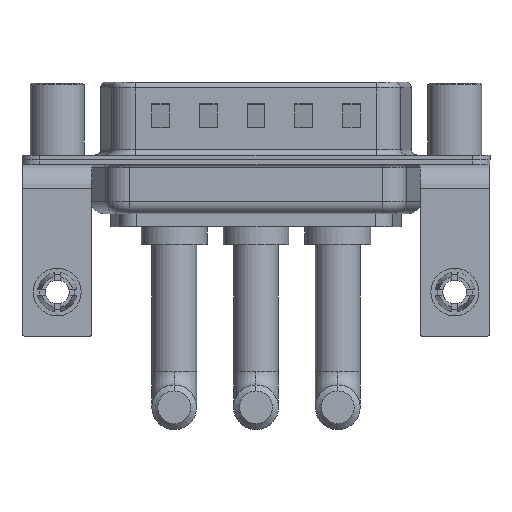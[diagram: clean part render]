
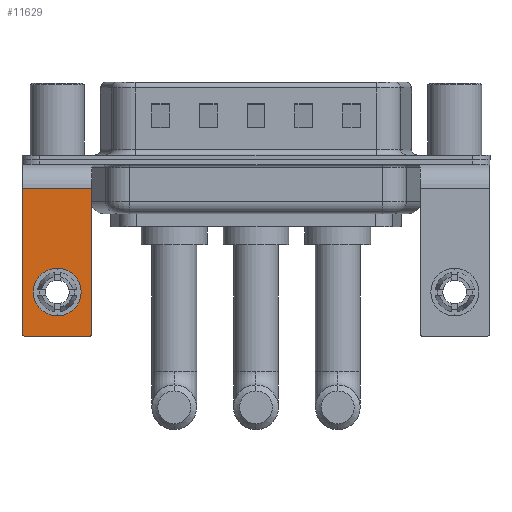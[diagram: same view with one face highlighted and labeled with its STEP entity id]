
A CAD part, front view. The second image highlights one B-rep face of the part: STEP entity #11629.
In plain terms, the highlighted planar face has unit normal (0, -1, 0).
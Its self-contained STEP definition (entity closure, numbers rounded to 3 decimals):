
#14 = ORIENTED_EDGE ( 'NONE', *, *, #4741, .T. ) ;
#195 = CARTESIAN_POINT ( 'NONE',  ( -2.9, -6.25, -2.4 ) ) ;
#734 = VERTEX_POINT ( 'NONE', #4127 ) ;
#1014 = DIRECTION ( 'NONE',  ( 0., 0., -1. ) ) ;
#1073 = CARTESIAN_POINT ( 'NONE',  ( 2.65, -6.25, -14.55 ) ) ;
#1187 = ORIENTED_EDGE ( 'NONE', *, *, #3510, .T. ) ;
#1225 = CIRCLE ( 'NONE', #14565, 2. ) ;
#1451 = EDGE_LOOP ( 'NONE', ( #7569, #5173, #8265, #14, #3821, #8792 ) ) ;
#1598 = DIRECTION ( 'NONE',  ( 0., 1., 0. ) ) ;
#1828 = AXIS2_PLACEMENT_3D ( 'NONE', #2882, #14920, #13556 ) ;
#2653 = EDGE_CURVE ( 'NONE', #9463, #10785, #3996, .T. ) ;
#2752 = VECTOR ( 'NONE', #1014, 1000. ) ;
#2882 = CARTESIAN_POINT ( 'NONE',  ( -2.65, -6.25, -14.55 ) ) ;
#2941 = ORIENTED_EDGE ( 'NONE', *, *, #8147, .T. ) ;
#3287 = DIRECTION ( 'NONE',  ( 0., 0., 1. ) ) ;
#3510 = EDGE_CURVE ( 'NONE', #17555, #18703, #1225, .T. ) ;
#3821 = ORIENTED_EDGE ( 'NONE', *, *, #11553, .F. ) ;
#3996 = CIRCLE ( 'NONE', #1828, 0.25 ) ;
#4127 = CARTESIAN_POINT ( 'NONE',  ( -2.9, -6.25, -2.4 ) ) ;
#4329 = AXIS2_PLACEMENT_3D ( 'NONE', #1073, #17310, #12748 ) ;
#4416 = DIRECTION ( 'NONE',  ( 0., 0., 1. ) ) ;
#4741 = EDGE_CURVE ( 'NONE', #13851, #15836, #6483, .T. ) ;
#5173 = ORIENTED_EDGE ( 'NONE', *, *, #2653, .T. ) ;
#5779 = CARTESIAN_POINT ( 'NONE',  ( 2.9, -6.25, -14.8 ) ) ;
#5844 = AXIS2_PLACEMENT_3D ( 'NONE', #8880, #1598, #4416 ) ;
#5859 = FACE_OUTER_BOUND ( 'NONE', #1451, .T. ) ;
#6004 = EDGE_CURVE ( 'NONE', #18560, #734, #10814, .T. ) ;
#6483 = CIRCLE ( 'NONE', #4329, 0.25 ) ;
#6920 = CARTESIAN_POINT ( 'NONE',  ( 2.9, -6.25, -2.4 ) ) ;
#7400 = VECTOR ( 'NONE', #16744, 1000. ) ;
#7569 = ORIENTED_EDGE ( 'NONE', *, *, #15988, .T. ) ;
#8147 = EDGE_CURVE ( 'NONE', #18703, #17555, #17874, .T. ) ;
#8236 = CARTESIAN_POINT ( 'NONE',  ( 0., -6.25, -11.07 ) ) ;
#8265 = ORIENTED_EDGE ( 'NONE', *, *, #9940, .F. ) ;
#8792 = ORIENTED_EDGE ( 'NONE', *, *, #6004, .T. ) ;
#8880 = CARTESIAN_POINT ( 'NONE',  ( 2.9, -6.25, -2.4 ) ) ;
#8922 = CARTESIAN_POINT ( 'NONE',  ( 0., -6.25, -11.07 ) ) ;
#9281 = CARTESIAN_POINT ( 'NONE',  ( 2.65, -6.25, -14.8 ) ) ;
#9353 = CARTESIAN_POINT ( 'NONE',  ( 2.9, -6.25, -2.4 ) ) ;
#9463 = VERTEX_POINT ( 'NONE', #18844 ) ;
#9489 = AXIS2_PLACEMENT_3D ( 'NONE', #8236, #17391, #9998 ) ;
#9940 = EDGE_CURVE ( 'NONE', #13851, #10785, #14349, .T. ) ;
#9998 = DIRECTION ( 'NONE',  ( 0., 0., 1. ) ) ;
#10776 = CARTESIAN_POINT ( 'NONE',  ( 0., -6.25, -9.07 ) ) ;
#10785 = VERTEX_POINT ( 'NONE', #13611 ) ;
#10814 = LINE ( 'NONE', #9353, #7400 ) ;
#11553 = EDGE_CURVE ( 'NONE', #18560, #15836, #17536, .T. ) ;
#11629 = ADVANCED_FACE ( 'NONE', ( #13359, #5859 ), #16283, .F. ) ;
#12126 = EDGE_LOOP ( 'NONE', ( #2941, #1187 ) ) ;
#12748 = DIRECTION ( 'NONE',  ( 0., 0., 1. ) ) ;
#12945 = CARTESIAN_POINT ( 'NONE',  ( 2.9, -6.25, -14.55 ) ) ;
#13359 = FACE_BOUND ( 'NONE', #12126, .T. ) ;
#13520 = DIRECTION ( 'NONE',  ( 0., 0., -1. ) ) ;
#13556 = DIRECTION ( 'NONE',  ( 0., 0., 1. ) ) ;
#13611 = CARTESIAN_POINT ( 'NONE',  ( -2.65, -6.25, -14.8 ) ) ;
#13851 = VERTEX_POINT ( 'NONE', #9281 ) ;
#14187 = VECTOR ( 'NONE', #17270, 1000. ) ;
#14349 = LINE ( 'NONE', #5779, #14187 ) ;
#14397 = CARTESIAN_POINT ( 'NONE',  ( 0., -6.25, -13.07 ) ) ;
#14565 = AXIS2_PLACEMENT_3D ( 'NONE', #8922, #15140, #3287 ) ;
#14920 = DIRECTION ( 'NONE',  ( 0., -1., 0. ) ) ;
#15140 = DIRECTION ( 'NONE',  ( 0., 1., 0. ) ) ;
#15811 = CARTESIAN_POINT ( 'NONE',  ( 2.9, -6.25, -2.4 ) ) ;
#15836 = VERTEX_POINT ( 'NONE', #12945 ) ;
#15988 = EDGE_CURVE ( 'NONE', #734, #9463, #18183, .T. ) ;
#16201 = VECTOR ( 'NONE', #13520, 1000. ) ;
#16283 = PLANE ( 'NONE',  #5844 ) ;
#16744 = DIRECTION ( 'NONE',  ( -1., 0., 0. ) ) ;
#17270 = DIRECTION ( 'NONE',  ( -1., 0., 0. ) ) ;
#17310 = DIRECTION ( 'NONE',  ( 0., -1., 0. ) ) ;
#17391 = DIRECTION ( 'NONE',  ( 0., 1., 0. ) ) ;
#17536 = LINE ( 'NONE', #15811, #2752 ) ;
#17555 = VERTEX_POINT ( 'NONE', #10776 ) ;
#17874 = CIRCLE ( 'NONE', #9489, 2. ) ;
#18183 = LINE ( 'NONE', #195, #16201 ) ;
#18560 = VERTEX_POINT ( 'NONE', #6920 ) ;
#18703 = VERTEX_POINT ( 'NONE', #14397 ) ;
#18844 = CARTESIAN_POINT ( 'NONE',  ( -2.9, -6.25, -14.55 ) ) ;
